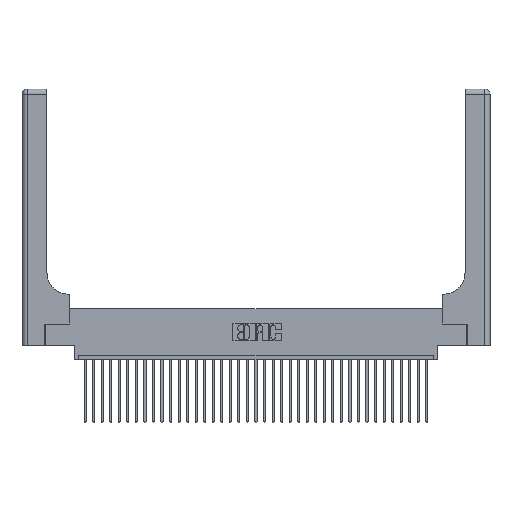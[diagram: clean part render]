
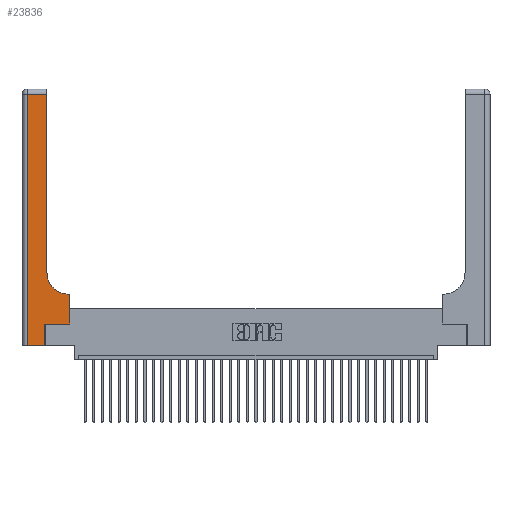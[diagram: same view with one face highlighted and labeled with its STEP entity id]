
A CAD part, top view. The second image highlights one B-rep face of the part: STEP entity #23836.
In plain terms, the highlighted planar face has unit normal (0, 0, 1).
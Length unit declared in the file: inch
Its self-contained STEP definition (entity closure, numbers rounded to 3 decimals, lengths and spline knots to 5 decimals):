
#399 = CARTESIAN_POINT ( 'NONE',  ( 0.2915, 0.6, 0.37 ) ) ;
#1192 = CARTESIAN_POINT ( 'NONE',  ( 0.06, 2.94, 0.37 ) ) ;
#1769 = DIRECTION ( 'NONE',  ( 0., 0., -1. ) ) ;
#1862 = LINE ( 'NONE', #4380, #10197 ) ;
#2061 = AXIS2_PLACEMENT_3D ( 'NONE', #32239, #35058, #30163 ) ;
#2256 = AXIS2_PLACEMENT_3D ( 'NONE', #13105, #1769, #7797 ) ;
#2812 = CARTESIAN_POINT ( 'NONE',  ( 0.269, 0., 0.37 ) ) ;
#3491 = EDGE_CURVE ( 'NONE', #29390, #8831, #16511, .T. ) ;
#4380 = CARTESIAN_POINT ( 'NONE',  ( 0., 2.94, 0.37 ) ) ;
#4878 = EDGE_CURVE ( 'NONE', #35610, #22352, #29084, .T. ) ;
#5945 = ORIENTED_EDGE ( 'NONE', *, *, #32594, .T. ) ;
#7672 = VERTEX_POINT ( 'NONE', #8139 ) ;
#7797 = DIRECTION ( 'NONE',  ( 1., 0., 0. ) ) ;
#7855 = CIRCLE ( 'NONE', #2256, 0.25 ) ;
#7948 = VERTEX_POINT ( 'NONE', #10086 ) ;
#8139 = CARTESIAN_POINT ( 'NONE',  ( 0.5585, 0.6, 0.37 ) ) ;
#8496 = VECTOR ( 'NONE', #25159, 39.37008 ) ;
#8831 = VERTEX_POINT ( 'NONE', #10683 ) ;
#10002 = VERTEX_POINT ( 'NONE', #24011 ) ;
#10086 = CARTESIAN_POINT ( 'NONE',  ( 0.2915, 2.94, 0.37 ) ) ;
#10197 = VECTOR ( 'NONE', #26316, 39.37008 ) ;
#10683 = CARTESIAN_POINT ( 'NONE',  ( 0.06, 0., 0.37 ) ) ;
#10754 = VERTEX_POINT ( 'NONE', #2812 ) ;
#10767 = CARTESIAN_POINT ( 'NONE',  ( 0.269, 0., 0.37 ) ) ;
#11425 = DIRECTION ( 'NONE',  ( 1., 0., 0. ) ) ;
#11730 = ORIENTED_EDGE ( 'NONE', *, *, #21819, .T. ) ;
#13105 = CARTESIAN_POINT ( 'NONE',  ( 0.5415, 0.85, 0.37 ) ) ;
#16198 = FACE_OUTER_BOUND ( 'NONE', #17213, .T. ) ;
#16511 = LINE ( 'NONE', #20253, #26111 ) ;
#16533 = CARTESIAN_POINT ( 'NONE',  ( 0.5585, 0.25, 0.37 ) ) ;
#16847 = DIRECTION ( 'NONE',  ( 0., -1., 0. ) ) ;
#17036 = EDGE_CURVE ( 'NONE', #10002, #7948, #26797, .T. ) ;
#17213 = EDGE_LOOP ( 'NONE', ( #32056, #5945, #34794, #11730, #23217, #31238, #26888, #33801, #19453 ) ) ;
#17479 = CARTESIAN_POINT ( 'NONE',  ( 0., 0., 0.37 ) ) ;
#17510 = DIRECTION ( 'NONE',  ( 0., 1., 0. ) ) ;
#18065 = VECTOR ( 'NONE', #30019, 39.37008 ) ;
#18893 = CARTESIAN_POINT ( 'NONE',  ( 0.269, 0.25, 0.37 ) ) ;
#19453 = ORIENTED_EDGE ( 'NONE', *, *, #22990, .T. ) ;
#20253 = CARTESIAN_POINT ( 'NONE',  ( 0.06, 3., 0.37 ) ) ;
#21183 = EDGE_CURVE ( 'NONE', #22352, #7672, #34817, .T. ) ;
#21678 = VERTEX_POINT ( 'NONE', #31733 ) ;
#21819 = EDGE_CURVE ( 'NONE', #8831, #10754, #35698, .T. ) ;
#21954 = CARTESIAN_POINT ( 'NONE',  ( 0.2915, 3., 0.37 ) ) ;
#22352 = VERTEX_POINT ( 'NONE', #35941 ) ;
#22990 = EDGE_CURVE ( 'NONE', #21678, #10002, #7855, .T. ) ;
#23217 = ORIENTED_EDGE ( 'NONE', *, *, #23377, .T. ) ;
#23377 = EDGE_CURVE ( 'NONE', #10754, #35610, #31028, .T. ) ;
#23836 = ADVANCED_FACE ( 'NONE', ( #16198 ), #28669, .F. ) ;
#24011 = CARTESIAN_POINT ( 'NONE',  ( 0.2915, 0.85, 0.37 ) ) ;
#25159 = DIRECTION ( 'NONE',  ( 0., 1., 0. ) ) ;
#26111 = VECTOR ( 'NONE', #16847, 39.37008 ) ;
#26316 = DIRECTION ( 'NONE',  ( -1., 0., 0. ) ) ;
#26341 = DIRECTION ( 'NONE',  ( -1., 0., 0. ) ) ;
#26469 = VECTOR ( 'NONE', #34460, 39.37008 ) ;
#26797 = LINE ( 'NONE', #21954, #18065 ) ;
#26888 = ORIENTED_EDGE ( 'NONE', *, *, #21183, .T. ) ;
#26989 = LINE ( 'NONE', #399, #35301 ) ;
#28669 = PLANE ( 'NONE',  #2061 ) ;
#29084 = LINE ( 'NONE', #30909, #30397 ) ;
#29390 = VERTEX_POINT ( 'NONE', #1192 ) ;
#30019 = DIRECTION ( 'NONE',  ( 0., 1., 0. ) ) ;
#30163 = DIRECTION ( 'NONE',  ( -1., 0., 0. ) ) ;
#30217 = VECTOR ( 'NONE', #17510, 39.37008 ) ;
#30397 = VECTOR ( 'NONE', #11425, 39.37008 ) ;
#30909 = CARTESIAN_POINT ( 'NONE',  ( 0.269, 0.25, 0.37 ) ) ;
#31028 = LINE ( 'NONE', #10767, #30217 ) ;
#31238 = ORIENTED_EDGE ( 'NONE', *, *, #4878, .T. ) ;
#31342 = EDGE_CURVE ( 'NONE', #7672, #21678, #26989, .T. ) ;
#31733 = CARTESIAN_POINT ( 'NONE',  ( 0.5415, 0.6, 0.37 ) ) ;
#32056 = ORIENTED_EDGE ( 'NONE', *, *, #17036, .T. ) ;
#32239 = CARTESIAN_POINT ( 'NONE',  ( 0., 3., 0.37 ) ) ;
#32594 = EDGE_CURVE ( 'NONE', #7948, #29390, #1862, .T. ) ;
#33801 = ORIENTED_EDGE ( 'NONE', *, *, #31342, .T. ) ;
#34460 = DIRECTION ( 'NONE',  ( 1., 0., 0. ) ) ;
#34794 = ORIENTED_EDGE ( 'NONE', *, *, #3491, .T. ) ;
#34817 = LINE ( 'NONE', #16533, #8496 ) ;
#35058 = DIRECTION ( 'NONE',  ( 0., 0., -1. ) ) ;
#35301 = VECTOR ( 'NONE', #26341, 39.37008 ) ;
#35610 = VERTEX_POINT ( 'NONE', #18893 ) ;
#35698 = LINE ( 'NONE', #17479, #26469 ) ;
#35941 = CARTESIAN_POINT ( 'NONE',  ( 0.5585, 0.25, 0.37 ) ) ;
